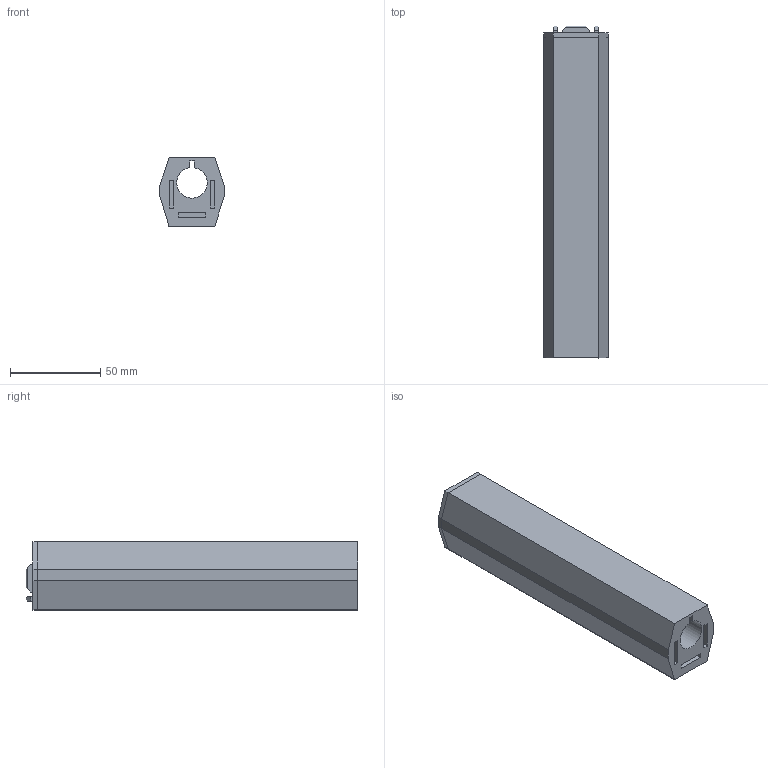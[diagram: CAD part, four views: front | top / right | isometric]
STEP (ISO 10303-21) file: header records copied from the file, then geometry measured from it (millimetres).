
FILE_DESCRIPTION(/* description */ (''),/* implementation_level */ '2;1');
FILE_NAME(/* name */ 'd878f440-f913-4d53-a883-f3277fcbb457.stp',/* time_stamp */ '2019-11-26T06:25:28+00:00',/* author */ (''),/* organization */ (''),/* preprocessor_version */ 'ST-DEVELOPER v18',/* originating_system */ 'Autodesk Translation Framework v8.12.0.6',/* authorisation */ '');
FILE_SCHEMA (('AUTOMOTIVE_DESIGN { 1 0 10303 214 3 1 1 }'));
Length unit declared in the file: inch
Products named in the file (1): Heritage Rough Rider - Fore End Extension
Bounding box: 35.56 x 184.15 x 38.1 mm (x, y, z)
Volume: 172293.3 mm3; surface area: 39606.3 mm2
Topology: 2 solids, 2 shells, 84 faces, 222 edges, 148 vertices
Faces by surface type: plane 82, cylinder 2
Entity records: 2604 total; most frequent: CARTESIAN_POINT 455, ORIENTED_EDGE 444, DIRECTION 396, EDGE_CURVE 222, LINE 218, VECTOR 218, VERTEX_POINT 148, EDGE_LOOP 100
